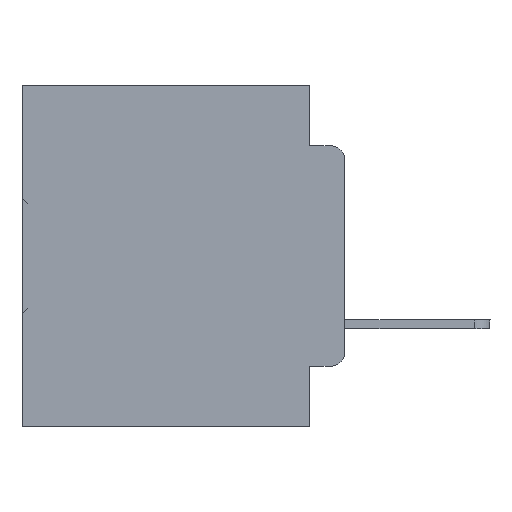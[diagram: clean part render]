
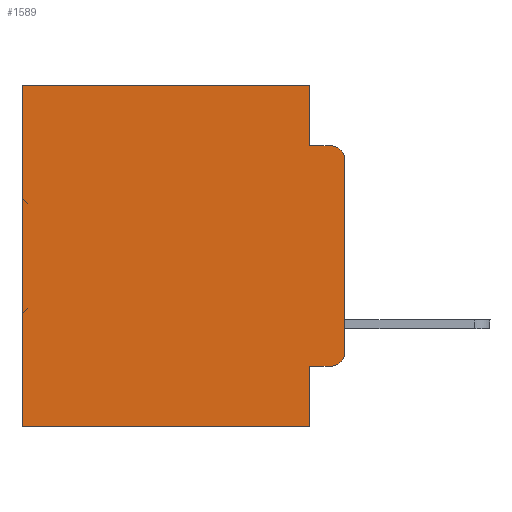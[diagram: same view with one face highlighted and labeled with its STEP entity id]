
A CAD part, left-side view. The second image highlights one B-rep face of the part: STEP entity #1589.
In plain terms, the highlighted planar face has unit normal (-1, 0, 0).
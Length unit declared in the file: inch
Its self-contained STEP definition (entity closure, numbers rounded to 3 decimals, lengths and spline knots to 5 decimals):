
#397 = CARTESIAN_POINT ( 'NONE',  ( 0.298, 0., 0. ) ) ;
#413 = LINE ( 'NONE', #18124, #33831 ) ;
#1589 = ADVANCED_FACE ( 'NONE', ( #1644 ), #33938, .F. ) ;
#1644 = FACE_OUTER_BOUND ( 'NONE', #14805, .T. ) ;
#2872 = VERTEX_POINT ( 'NONE', #17700 ) ;
#2941 = LINE ( 'NONE', #33659, #31976 ) ;
#3082 = DIRECTION ( 'NONE',  ( 1., 0., 0. ) ) ;
#4411 = VERTEX_POINT ( 'NONE', #6022 ) ;
#5339 = VERTEX_POINT ( 'NONE', #27383 ) ;
#5909 = CARTESIAN_POINT ( 'NONE',  ( 0.298, 0.02, -0.1085 ) ) ;
#6022 = CARTESIAN_POINT ( 'NONE',  ( 0.298, 0.051, -0.0885 ) ) ;
#6066 = CIRCLE ( 'NONE', #18076, 0.02 ) ;
#6529 = DIRECTION ( 'NONE',  ( 0., 0., -1. ) ) ;
#6743 = DIRECTION ( 'NONE',  ( 0., -1., 0. ) ) ;
#7213 = LINE ( 'NONE', #28485, #21300 ) ;
#7583 = CARTESIAN_POINT ( 'NONE',  ( 0.298, 0.051, 0. ) ) ;
#7697 = VERTEX_POINT ( 'NONE', #7583 ) ;
#7851 = CARTESIAN_POINT ( 'NONE',  ( 0.298, 0.02, -0.4115 ) ) ;
#9160 = EDGE_CURVE ( 'NONE', #24739, #5339, #7213, .T. ) ;
#9820 = ORIENTED_EDGE ( 'NONE', *, *, #9160, .F. ) ;
#10064 = CARTESIAN_POINT ( 'NONE',  ( 0.298, 0.051, -0.4115 ) ) ;
#10108 = VECTOR ( 'NONE', #18649, 39.37008 ) ;
#10137 = ORIENTED_EDGE ( 'NONE', *, *, #24446, .T. ) ;
#10329 = LINE ( 'NONE', #20418, #21341 ) ;
#10649 = DIRECTION ( 'NONE',  ( 0., -1., 0. ) ) ;
#11175 = DIRECTION ( 'NONE',  ( 0., 0., -1. ) ) ;
#12149 = DIRECTION ( 'NONE',  ( 0., 1., 0. ) ) ;
#12329 = EDGE_CURVE ( 'NONE', #21361, #34733, #6066, .T. ) ;
#12556 = CARTESIAN_POINT ( 'NONE',  ( 0.298, 0., -0.3915 ) ) ;
#14110 = AXIS2_PLACEMENT_3D ( 'NONE', #5909, #33948, #19916 ) ;
#14212 = CARTESIAN_POINT ( 'NONE',  ( 0.298, 0.02, -0.0885 ) ) ;
#14805 = EDGE_LOOP ( 'NONE', ( #28436, #10137, #15947, #17556, #16184, #36426, #9820, #23612, #23845, #25780 ) ) ;
#15227 = CARTESIAN_POINT ( 'NONE',  ( 0.298, 0., 0. ) ) ;
#15947 = ORIENTED_EDGE ( 'NONE', *, *, #32177, .F. ) ;
#16184 = ORIENTED_EDGE ( 'NONE', *, *, #31239, .T. ) ;
#16597 = VECTOR ( 'NONE', #22392, 39.37008 ) ;
#16683 = EDGE_CURVE ( 'NONE', #33329, #5339, #10329, .T. ) ;
#16816 = DIRECTION ( 'NONE',  ( 0., 0., -1. ) ) ;
#17149 = VERTEX_POINT ( 'NONE', #14212 ) ;
#17556 = ORIENTED_EDGE ( 'NONE', *, *, #30017, .F. ) ;
#17700 = CARTESIAN_POINT ( 'NONE',  ( 0.298, 0.051, -0.4115 ) ) ;
#18076 = AXIS2_PLACEMENT_3D ( 'NONE', #22586, #25291, #27875 ) ;
#18124 = CARTESIAN_POINT ( 'NONE',  ( 0.298, 0., 0. ) ) ;
#18312 = CARTESIAN_POINT ( 'NONE',  ( 0.298, 0.051, -0.5 ) ) ;
#18649 = DIRECTION ( 'NONE',  ( 0., 0., -1. ) ) ;
#19916 = DIRECTION ( 'NONE',  ( 0., 0., -1. ) ) ;
#20418 = CARTESIAN_POINT ( 'NONE',  ( 0.298, 0.473, 0. ) ) ;
#21095 = EDGE_CURVE ( 'NONE', #2872, #24739, #28019, .T. ) ;
#21116 = AXIS2_PLACEMENT_3D ( 'NONE', #397, #3082, #11175 ) ;
#21300 = VECTOR ( 'NONE', #12149, 39.37008 ) ;
#21341 = VECTOR ( 'NONE', #6529, 39.37008 ) ;
#21361 = VERTEX_POINT ( 'NONE', #7851 ) ;
#21856 = CARTESIAN_POINT ( 'NONE',  ( 0.298, 0.051, -0.0885 ) ) ;
#21895 = CARTESIAN_POINT ( 'NONE',  ( 0.298, 0.473, 0. ) ) ;
#21997 = LINE ( 'NONE', #15227, #10108 ) ;
#22392 = DIRECTION ( 'NONE',  ( 0., 0., -1. ) ) ;
#22586 = CARTESIAN_POINT ( 'NONE',  ( 0.298, 0.02, -0.3915 ) ) ;
#23612 = ORIENTED_EDGE ( 'NONE', *, *, #21095, .F. ) ;
#23845 = ORIENTED_EDGE ( 'NONE', *, *, #35552, .T. ) ;
#24446 = EDGE_CURVE ( 'NONE', #35032, #17149, #31703, .T. ) ;
#24739 = VERTEX_POINT ( 'NONE', #18312 ) ;
#24930 = LINE ( 'NONE', #21856, #25392 ) ;
#25088 = CARTESIAN_POINT ( 'NONE',  ( 0.298, 0., -0.1085 ) ) ;
#25291 = DIRECTION ( 'NONE',  ( -1., 0., 0. ) ) ;
#25392 = VECTOR ( 'NONE', #10649, 39.37008 ) ;
#25780 = ORIENTED_EDGE ( 'NONE', *, *, #12329, .T. ) ;
#26496 = LINE ( 'NONE', #10064, #31319 ) ;
#27383 = CARTESIAN_POINT ( 'NONE',  ( 0.298, 0.473, -0.5 ) ) ;
#27875 = DIRECTION ( 'NONE',  ( 0., 0., -1. ) ) ;
#28019 = LINE ( 'NONE', #33574, #16597 ) ;
#28427 = EDGE_CURVE ( 'NONE', #35032, #34733, #21997, .T. ) ;
#28436 = ORIENTED_EDGE ( 'NONE', *, *, #28427, .F. ) ;
#28485 = CARTESIAN_POINT ( 'NONE',  ( 0.298, 0., -0.5 ) ) ;
#30017 = EDGE_CURVE ( 'NONE', #7697, #4411, #2941, .T. ) ;
#30920 = DIRECTION ( 'NONE',  ( 0., 1., 0. ) ) ;
#31239 = EDGE_CURVE ( 'NONE', #7697, #33329, #413, .T. ) ;
#31319 = VECTOR ( 'NONE', #6743, 39.37008 ) ;
#31703 = CIRCLE ( 'NONE', #14110, 0.02 ) ;
#31976 = VECTOR ( 'NONE', #16816, 39.37008 ) ;
#32177 = EDGE_CURVE ( 'NONE', #4411, #17149, #24930, .T. ) ;
#33329 = VERTEX_POINT ( 'NONE', #21895 ) ;
#33574 = CARTESIAN_POINT ( 'NONE',  ( 0.298, 0.051, 0. ) ) ;
#33659 = CARTESIAN_POINT ( 'NONE',  ( 0.298, 0.051, 0. ) ) ;
#33831 = VECTOR ( 'NONE', #30920, 39.37008 ) ;
#33938 = PLANE ( 'NONE',  #21116 ) ;
#33948 = DIRECTION ( 'NONE',  ( -1., 0., 0. ) ) ;
#34733 = VERTEX_POINT ( 'NONE', #12556 ) ;
#35032 = VERTEX_POINT ( 'NONE', #25088 ) ;
#35552 = EDGE_CURVE ( 'NONE', #2872, #21361, #26496, .T. ) ;
#36426 = ORIENTED_EDGE ( 'NONE', *, *, #16683, .T. ) ;
